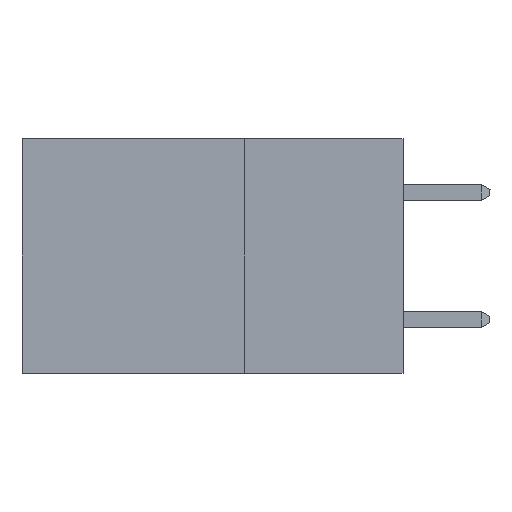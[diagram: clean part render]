
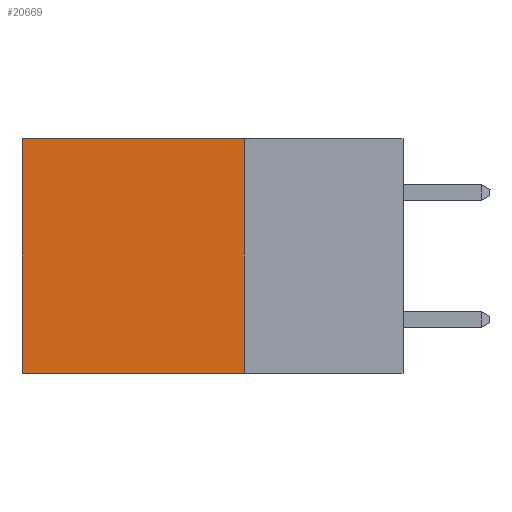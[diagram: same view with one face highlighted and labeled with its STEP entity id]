
A CAD part, left-side view. The second image highlights one B-rep face of the part: STEP entity #20669.
In plain terms, the highlighted planar face has unit normal (-1, 0, 0).
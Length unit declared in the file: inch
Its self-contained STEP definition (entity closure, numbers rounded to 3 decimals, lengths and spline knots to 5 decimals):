
#231 = DIRECTION ( 'NONE',  ( 0., 0., -1. ) ) ;
#1100 = VERTEX_POINT ( 'NONE', #18655 ) ;
#1266 = VERTEX_POINT ( 'NONE', #13842 ) ;
#1370 = EDGE_CURVE ( 'NONE', #7439, #1100, #18589, .T. ) ;
#1545 = EDGE_CURVE ( 'NONE', #7439, #2671, #15256, .T. ) ;
#1615 = CARTESIAN_POINT ( 'NONE',  ( 0.2875, 0.25, 0. ) ) ;
#1812 = CARTESIAN_POINT ( 'NONE',  ( 0.2875, 0.25, 0. ) ) ;
#2101 = ORIENTED_EDGE ( 'NONE', *, *, #9872, .F. ) ;
#2671 = VERTEX_POINT ( 'NONE', #12230 ) ;
#4109 = PLANE ( 'NONE',  #17927 ) ;
#4266 = EDGE_LOOP ( 'NONE', ( #11163, #2101, #21536, #21787 ) ) ;
#5476 = VECTOR ( 'NONE', #12356, 39.37008 ) ;
#7360 = CARTESIAN_POINT ( 'NONE',  ( 0.2875, 0.6, 0. ) ) ;
#7439 = VERTEX_POINT ( 'NONE', #1812 ) ;
#7449 = DIRECTION ( 'NONE',  ( 0., 1., 0. ) ) ;
#7748 = DIRECTION ( 'NONE',  ( 1., 0., 0. ) ) ;
#7762 = CARTESIAN_POINT ( 'NONE',  ( 0.2875, 0.25, -0.37 ) ) ;
#7853 = VECTOR ( 'NONE', #18410, 39.37008 ) ;
#8704 = FACE_OUTER_BOUND ( 'NONE', #4266, .T. ) ;
#8859 = LINE ( 'NONE', #7360, #17777 ) ;
#9872 = EDGE_CURVE ( 'NONE', #1100, #1266, #12028, .T. ) ;
#10512 = VECTOR ( 'NONE', #7449, 39.37008 ) ;
#11163 = ORIENTED_EDGE ( 'NONE', *, *, #17553, .T. ) ;
#12028 = LINE ( 'NONE', #7762, #7853 ) ;
#12230 = CARTESIAN_POINT ( 'NONE',  ( 0.2875, 0.6, 0. ) ) ;
#12356 = DIRECTION ( 'NONE',  ( 0., 0., -1. ) ) ;
#13842 = CARTESIAN_POINT ( 'NONE',  ( 0.2875, 0.6, -0.37 ) ) ;
#15256 = LINE ( 'NONE', #21653, #10512 ) ;
#17553 = EDGE_CURVE ( 'NONE', #2671, #1266, #8859, .T. ) ;
#17777 = VECTOR ( 'NONE', #231, 39.37008 ) ;
#17927 = AXIS2_PLACEMENT_3D ( 'NONE', #18398, #7748, #20156 ) ;
#18398 = CARTESIAN_POINT ( 'NONE',  ( 0.2875, 0.25, 0. ) ) ;
#18410 = DIRECTION ( 'NONE',  ( 0., 1., 0. ) ) ;
#18589 = LINE ( 'NONE', #1615, #5476 ) ;
#18655 = CARTESIAN_POINT ( 'NONE',  ( 0.2875, 0.25, -0.37 ) ) ;
#20156 = DIRECTION ( 'NONE',  ( 0., 0., -1. ) ) ;
#20669 = ADVANCED_FACE ( 'NONE', ( #8704 ), #4109, .F. ) ;
#21536 = ORIENTED_EDGE ( 'NONE', *, *, #1370, .F. ) ;
#21653 = CARTESIAN_POINT ( 'NONE',  ( 0.2875, 0.25, 0. ) ) ;
#21787 = ORIENTED_EDGE ( 'NONE', *, *, #1545, .T. ) ;
